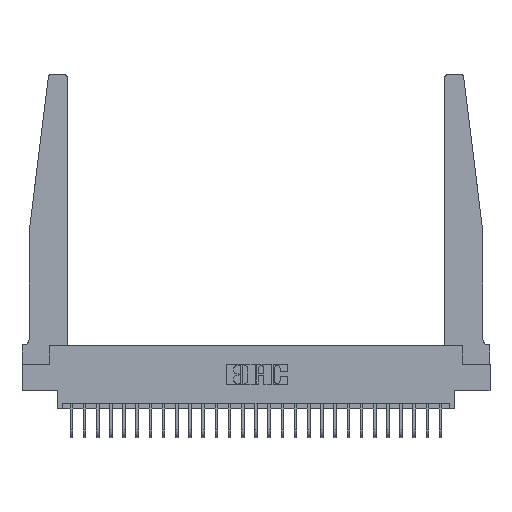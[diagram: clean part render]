
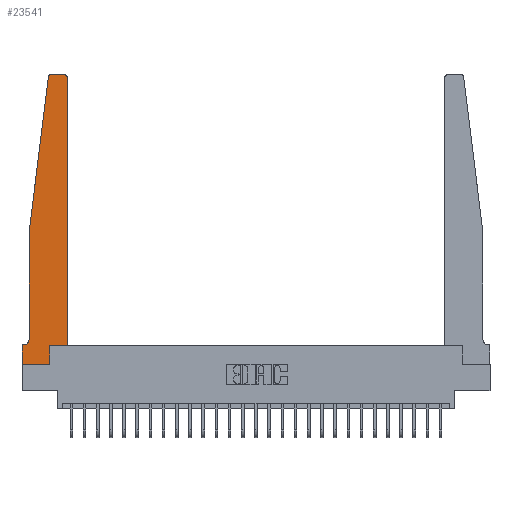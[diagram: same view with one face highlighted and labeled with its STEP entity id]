
A CAD part, top view. The second image highlights one B-rep face of the part: STEP entity #23541.
In plain terms, the highlighted planar face has unit normal (0, 0, 1).
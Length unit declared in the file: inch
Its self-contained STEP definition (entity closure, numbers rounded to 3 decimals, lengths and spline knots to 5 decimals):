
#694 = AXIS2_PLACEMENT_3D ( 'NONE', #21529, #10173, #23394 ) ;
#840 = DIRECTION ( 'NONE',  ( 0., 0., -1. ) ) ;
#874 = AXIS2_PLACEMENT_3D ( 'NONE', #18970, #7587, #20852 ) ;
#1052 = CARTESIAN_POINT ( 'NONE',  ( 0.425, 0.18, 0.37 ) ) ;
#1429 = DIRECTION ( 'NONE',  ( 0., 0., 1. ) ) ;
#1622 = VERTEX_POINT ( 'NONE', #12568 ) ;
#2478 = LINE ( 'NONE', #22898, #21557 ) ;
#2485 = VECTOR ( 'NONE', #10682, 39.37008 ) ;
#2790 = DIRECTION ( 'NONE',  ( -1., 0., 0. ) ) ;
#3236 = VERTEX_POINT ( 'NONE', #13465 ) ;
#3328 = CARTESIAN_POINT ( 'NONE',  ( 0., 0.1875, 0.37 ) ) ;
#3399 = CARTESIAN_POINT ( 'NONE',  ( 0., 0.1875, 0.37 ) ) ;
#3880 = LINE ( 'NONE', #4596, #12849 ) ;
#3904 = CARTESIAN_POINT ( 'NONE',  ( 0.425, 0.18, 0.37 ) ) ;
#4596 = CARTESIAN_POINT ( 'NONE',  ( 0., 0., 0.37 ) ) ;
#4825 = DIRECTION ( 'NONE',  ( -0.122, -0.992, 0. ) ) ;
#5729 = VECTOR ( 'NONE', #14317, 39.37008 ) ;
#6028 = ORIENTED_EDGE ( 'NONE', *, *, #22022, .T. ) ;
#6037 = CARTESIAN_POINT ( 'NONE',  ( 0.395, 2.75, 0.37 ) ) ;
#6084 = EDGE_CURVE ( 'NONE', #21129, #1622, #3880, .T. ) ;
#6156 = CIRCLE ( 'NONE', #874, 0.03 ) ;
#6462 = VERTEX_POINT ( 'NONE', #8208 ) ;
#7003 = ORIENTED_EDGE ( 'NONE', *, *, #12590, .T. ) ;
#7347 = VECTOR ( 'NONE', #2790, 39.37008 ) ;
#7415 = CARTESIAN_POINT ( 'NONE',  ( 0.27653, 2.75, 0.37 ) ) ;
#7496 = VERTEX_POINT ( 'NONE', #7415 ) ;
#7587 = DIRECTION ( 'NONE',  ( 0., 0., 1. ) ) ;
#7609 = VECTOR ( 'NONE', #11437, 39.37008 ) ;
#7762 = DIRECTION ( 'NONE',  ( 0., 1., 0. ) ) ;
#8208 = CARTESIAN_POINT ( 'NONE',  ( 0.015, 0.1875, 0.37 ) ) ;
#8212 = LINE ( 'NONE', #24607, #7609 ) ;
#8331 = CARTESIAN_POINT ( 'NONE',  ( 0.425, 0.18, 0.37 ) ) ;
#8622 = CIRCLE ( 'NONE', #18830, 0.05 ) ;
#9124 = VERTEX_POINT ( 'NONE', #11660 ) ;
#9151 = VERTEX_POINT ( 'NONE', #6037 ) ;
#9284 = ORIENTED_EDGE ( 'NONE', *, *, #24050, .T. ) ;
#9408 = VERTEX_POINT ( 'NONE', #16193 ) ;
#10173 = DIRECTION ( 'NONE',  ( 0., 0., 1. ) ) ;
#10232 = CARTESIAN_POINT ( 'NONE',  ( 0.065, 0.2375, 0.37 ) ) ;
#10371 = EDGE_CURVE ( 'NONE', #9151, #7496, #8212, .T. ) ;
#10409 = EDGE_CURVE ( 'NONE', #9124, #22010, #2478, .T. ) ;
#10682 = DIRECTION ( 'NONE',  ( 0., 1., 0. ) ) ;
#10962 = PLANE ( 'NONE',  #12658 ) ;
#11308 = VERTEX_POINT ( 'NONE', #10232 ) ;
#11353 = VECTOR ( 'NONE', #17265, 39.37008 ) ;
#11420 = EDGE_CURVE ( 'NONE', #1622, #9124, #15894, .T. ) ;
#11437 = DIRECTION ( 'NONE',  ( -1., 0., 0. ) ) ;
#11660 = CARTESIAN_POINT ( 'NONE',  ( 0.2605, 0., 0.37 ) ) ;
#11680 = ORIENTED_EDGE ( 'NONE', *, *, #17444, .T. ) ;
#11836 = LINE ( 'NONE', #14271, #7347 ) ;
#12240 = CARTESIAN_POINT ( 'NONE',  ( 0.2605, 0.18, 0.37 ) ) ;
#12299 = VECTOR ( 'NONE', #23002, 39.37008 ) ;
#12310 = DIRECTION ( 'NONE',  ( 0., -1., 0. ) ) ;
#12405 = CARTESIAN_POINT ( 'NONE',  ( 0.015, 0.2375, 0.37 ) ) ;
#12568 = CARTESIAN_POINT ( 'NONE',  ( 0., 0., 0.37 ) ) ;
#12590 = EDGE_CURVE ( 'NONE', #6462, #21129, #11836, .T. ) ;
#12658 = AXIS2_PLACEMENT_3D ( 'NONE', #3328, #1429, #14875 ) ;
#12799 = VECTOR ( 'NONE', #4825, 39.37008 ) ;
#12849 = VECTOR ( 'NONE', #12310, 39.37008 ) ;
#12851 = EDGE_CURVE ( 'NONE', #19738, #9151, #6156, .T. ) ;
#13088 = ORIENTED_EDGE ( 'NONE', *, *, #22748, .T. ) ;
#13465 = CARTESIAN_POINT ( 'NONE',  ( 0.24675, 2.72367, 0.37 ) ) ;
#14271 = CARTESIAN_POINT ( 'NONE',  ( 0.065, 0.1875, 0.37 ) ) ;
#14317 = DIRECTION ( 'NONE',  ( 1., 0., 0. ) ) ;
#14320 = DIRECTION ( 'NONE',  ( -1., 0., 0. ) ) ;
#14475 = ORIENTED_EDGE ( 'NONE', *, *, #12851, .T. ) ;
#14875 = DIRECTION ( 'NONE',  ( 1., 0., 0. ) ) ;
#15323 = ORIENTED_EDGE ( 'NONE', *, *, #21347, .T. ) ;
#15894 = LINE ( 'NONE', #16206, #5729 ) ;
#16193 = CARTESIAN_POINT ( 'NONE',  ( 0.065, 1.25, 0.37 ) ) ;
#16206 = CARTESIAN_POINT ( 'NONE',  ( 0., 0., 0.37 ) ) ;
#16614 = CIRCLE ( 'NONE', #694, 0.03 ) ;
#17265 = DIRECTION ( 'NONE',  ( 1., 0., 0. ) ) ;
#17444 = EDGE_CURVE ( 'NONE', #3236, #9408, #22844, .T. ) ;
#17524 = ORIENTED_EDGE ( 'NONE', *, *, #10409, .T. ) ;
#18518 = LINE ( 'NONE', #21140, #12299 ) ;
#18830 = AXIS2_PLACEMENT_3D ( 'NONE', #12405, #840, #14320 ) ;
#18941 = FACE_OUTER_BOUND ( 'NONE', #22250, .T. ) ;
#18970 = CARTESIAN_POINT ( 'NONE',  ( 0.395, 2.72, 0.37 ) ) ;
#19513 = EDGE_CURVE ( 'NONE', #9408, #11308, #18518, .T. ) ;
#19738 = VERTEX_POINT ( 'NONE', #22008 ) ;
#20095 = ORIENTED_EDGE ( 'NONE', *, *, #10371, .T. ) ;
#20207 = VERTEX_POINT ( 'NONE', #8331 ) ;
#20852 = DIRECTION ( 'NONE',  ( 1., 0., 0. ) ) ;
#21129 = VERTEX_POINT ( 'NONE', #3399 ) ;
#21140 = CARTESIAN_POINT ( 'NONE',  ( 0.065, 1.25, 0.37 ) ) ;
#21347 = EDGE_CURVE ( 'NONE', #22010, #20207, #21995, .T. ) ;
#21529 = CARTESIAN_POINT ( 'NONE',  ( 0.27653, 2.72, 0.37 ) ) ;
#21557 = VECTOR ( 'NONE', #7762, 39.37008 ) ;
#21884 = CARTESIAN_POINT ( 'NONE',  ( 0.065, 1.25, 0.37 ) ) ;
#21917 = ORIENTED_EDGE ( 'NONE', *, *, #11420, .T. ) ;
#21995 = LINE ( 'NONE', #3904, #11353 ) ;
#22008 = CARTESIAN_POINT ( 'NONE',  ( 0.425, 2.72, 0.37 ) ) ;
#22010 = VERTEX_POINT ( 'NONE', #12240 ) ;
#22022 = EDGE_CURVE ( 'NONE', #11308, #6462, #8622, .T. ) ;
#22250 = EDGE_LOOP ( 'NONE', ( #20095, #13088, #11680, #22406, #6028, #7003, #23111, #21917, #17524, #15323, #9284, #14475 ) ) ;
#22406 = ORIENTED_EDGE ( 'NONE', *, *, #19513, .T. ) ;
#22716 = LINE ( 'NONE', #1052, #2485 ) ;
#22748 = EDGE_CURVE ( 'NONE', #7496, #3236, #16614, .T. ) ;
#22844 = LINE ( 'NONE', #21884, #12799 ) ;
#22898 = CARTESIAN_POINT ( 'NONE',  ( 0.2605, 0.18, 0.37 ) ) ;
#23002 = DIRECTION ( 'NONE',  ( 0., -1., 0. ) ) ;
#23111 = ORIENTED_EDGE ( 'NONE', *, *, #6084, .T. ) ;
#23394 = DIRECTION ( 'NONE',  ( 1., 0., 0. ) ) ;
#23541 = ADVANCED_FACE ( 'NONE', ( #18941 ), #10962, .T. ) ;
#24050 = EDGE_CURVE ( 'NONE', #20207, #19738, #22716, .T. ) ;
#24607 = CARTESIAN_POINT ( 'NONE',  ( 0.25, 2.75, 0.37 ) ) ;
